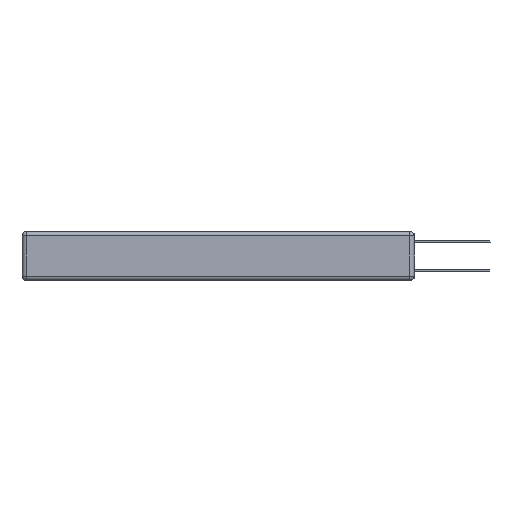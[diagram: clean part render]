
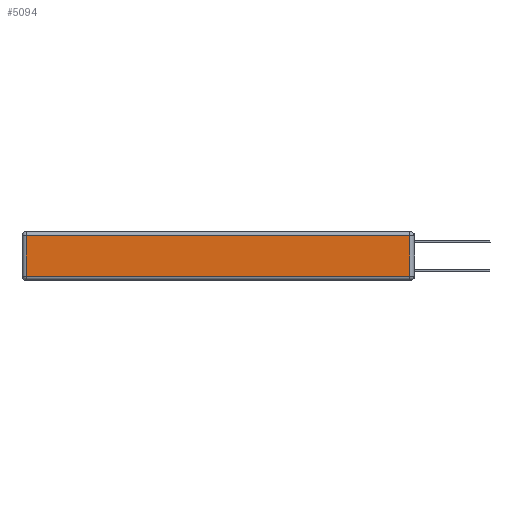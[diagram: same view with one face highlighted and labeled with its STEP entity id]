
A CAD part, left-side view. The second image highlights one B-rep face of the part: STEP entity #5094.
In plain terms, the highlighted planar face has unit normal (-1, 0, 0).
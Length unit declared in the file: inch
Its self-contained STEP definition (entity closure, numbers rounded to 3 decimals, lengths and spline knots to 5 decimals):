
#623 = VERTEX_POINT ( 'NONE', #7986 ) ;
#798 = LINE ( 'NONE', #13729, #4286 ) ;
#1538 = DIRECTION ( 'NONE',  ( -1., 0., 0. ) ) ;
#1667 = DIRECTION ( 'NONE',  ( 0., 0., 1. ) ) ;
#1979 = ORIENTED_EDGE ( 'NONE', *, *, #4706, .T. ) ;
#2028 = DIRECTION ( 'NONE',  ( 0., 0., -1. ) ) ;
#2217 = ORIENTED_EDGE ( 'NONE', *, *, #11152, .T. ) ;
#2266 = EDGE_LOOP ( 'NONE', ( #12618, #1979, #5619, #2217 ) ) ;
#2752 = DIRECTION ( 'NONE',  ( 0., 0., 1. ) ) ;
#4081 = CARTESIAN_POINT ( 'NONE',  ( 0., 0., -0.313 ) ) ;
#4286 = VECTOR ( 'NONE', #2028, 39.37008 ) ;
#4329 = EDGE_CURVE ( 'NONE', #13584, #13415, #4946, .T. ) ;
#4623 = EDGE_CURVE ( 'NONE', #623, #15453, #16645, .T. ) ;
#4706 = EDGE_CURVE ( 'NONE', #15453, #13584, #13817, .T. ) ;
#4946 = LINE ( 'NONE', #16918, #12447 ) ;
#5094 = ADVANCED_FACE ( 'NONE', ( #14487 ), #7563, .T. ) ;
#5619 = ORIENTED_EDGE ( 'NONE', *, *, #4329, .T. ) ;
#7563 = PLANE ( 'NONE',  #12843 ) ;
#7835 = CARTESIAN_POINT ( 'NONE',  ( 0., 0.03, -0.03 ) ) ;
#7838 = DIRECTION ( 'NONE',  ( 0., 1., 0. ) ) ;
#7986 = CARTESIAN_POINT ( 'NONE',  ( 0., 2.72, -0.313 ) ) ;
#9676 = VECTOR ( 'NONE', #11500, 39.37008 ) ;
#10717 = CARTESIAN_POINT ( 'NONE',  ( 0., 0., -0.343 ) ) ;
#11152 = EDGE_CURVE ( 'NONE', #13415, #623, #798, .T. ) ;
#11500 = DIRECTION ( 'NONE',  ( 0., -1., 0. ) ) ;
#11862 = CARTESIAN_POINT ( 'NONE',  ( 0., 0.03, -0.343 ) ) ;
#12447 = VECTOR ( 'NONE', #7838, 39.37008 ) ;
#12618 = ORIENTED_EDGE ( 'NONE', *, *, #4623, .T. ) ;
#12843 = AXIS2_PLACEMENT_3D ( 'NONE', #10717, #1538, #1667 ) ;
#13415 = VERTEX_POINT ( 'NONE', #16193 ) ;
#13584 = VERTEX_POINT ( 'NONE', #7835 ) ;
#13729 = CARTESIAN_POINT ( 'NONE',  ( 0., 2.72, -0.343 ) ) ;
#13817 = LINE ( 'NONE', #11862, #16861 ) ;
#13959 = CARTESIAN_POINT ( 'NONE',  ( 0., 0.03, -0.313 ) ) ;
#14487 = FACE_OUTER_BOUND ( 'NONE', #2266, .T. ) ;
#15453 = VERTEX_POINT ( 'NONE', #13959 ) ;
#16193 = CARTESIAN_POINT ( 'NONE',  ( 0., 2.72, -0.03 ) ) ;
#16645 = LINE ( 'NONE', #4081, #9676 ) ;
#16861 = VECTOR ( 'NONE', #2752, 39.37008 ) ;
#16918 = CARTESIAN_POINT ( 'NONE',  ( 0., 2.75, -0.03 ) ) ;
